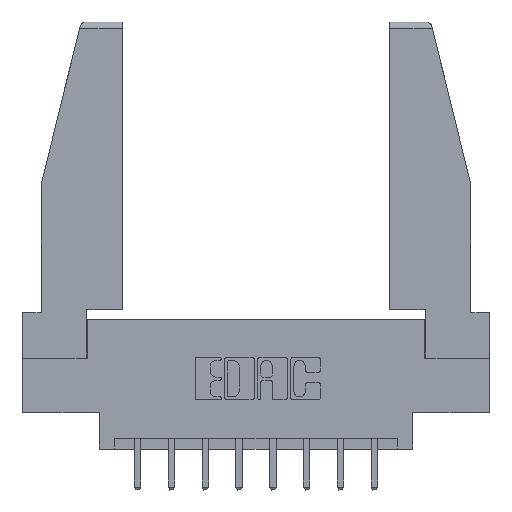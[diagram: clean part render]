
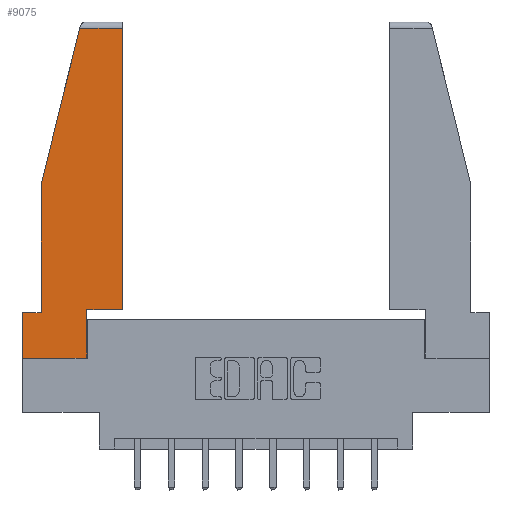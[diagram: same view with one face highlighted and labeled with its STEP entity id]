
A CAD part, top view. The second image highlights one B-rep face of the part: STEP entity #9075.
In plain terms, the highlighted planar face has unit normal (0, 0, 1).
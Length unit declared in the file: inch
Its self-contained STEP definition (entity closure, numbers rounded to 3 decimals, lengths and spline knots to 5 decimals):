
#29 = VERTEX_POINT ( 'NONE', #10967 ) ;
#134 = DIRECTION ( 'NONE',  ( 0., -1., 0. ) ) ;
#291 = ORIENTED_EDGE ( 'NONE', *, *, #1685, .T. ) ;
#474 = LINE ( 'NONE', #6805, #2551 ) ;
#528 = VERTEX_POINT ( 'NONE', #4427 ) ;
#845 = VECTOR ( 'NONE', #8664, 39.37008 ) ;
#1119 = VECTOR ( 'NONE', #6566, 39.37008 ) ;
#1157 = DIRECTION ( 'NONE',  ( 0., 1., 0. ) ) ;
#1420 = VERTEX_POINT ( 'NONE', #6144 ) ;
#1426 = VECTOR ( 'NONE', #8244, 39.37008 ) ;
#1634 = ORIENTED_EDGE ( 'NONE', *, *, #9630, .T. ) ;
#1685 = EDGE_CURVE ( 'NONE', #1420, #528, #12575, .T. ) ;
#1731 = EDGE_CURVE ( 'NONE', #9567, #5478, #4646, .T. ) ;
#1745 = CARTESIAN_POINT ( 'NONE',  ( 0., 0.21, 0. ) ) ;
#2107 = DIRECTION ( 'NONE',  ( 0., 0., 1. ) ) ;
#2132 = LINE ( 'NONE', #12660, #845 ) ;
#2157 = ORIENTED_EDGE ( 'NONE', *, *, #1731, .T. ) ;
#2300 = DIRECTION ( 'NONE',  ( 0., 1., 0. ) ) ;
#2551 = VECTOR ( 'NONE', #7887, 39.37008 ) ;
#2657 = EDGE_CURVE ( 'NONE', #5478, #3469, #474, .T. ) ;
#2764 = ORIENTED_EDGE ( 'NONE', *, *, #2977, .T. ) ;
#2782 = LINE ( 'NONE', #5480, #9214 ) ;
#2977 = EDGE_CURVE ( 'NONE', #3469, #12307, #10913, .T. ) ;
#3406 = LINE ( 'NONE', #8216, #6632 ) ;
#3469 = VERTEX_POINT ( 'NONE', #1745 ) ;
#4027 = PLANE ( 'NONE',  #12430 ) ;
#4427 = CARTESIAN_POINT ( 'NONE',  ( 0.297, 0.223, 0. ) ) ;
#4522 = CARTESIAN_POINT ( 'NONE',  ( 0.086, 0.8, 0. ) ) ;
#4646 = LINE ( 'NONE', #4522, #1119 ) ;
#4932 = ORIENTED_EDGE ( 'NONE', *, *, #8608, .T. ) ;
#5478 = VERTEX_POINT ( 'NONE', #9220 ) ;
#5480 = CARTESIAN_POINT ( 'NONE',  ( 0.271, 1.55, 0. ) ) ;
#5542 = CARTESIAN_POINT ( 'NONE',  ( 0.086, 0.8, 0. ) ) ;
#5574 = CARTESIAN_POINT ( 'NONE',  ( 0.461, 0.223, 0. ) ) ;
#5576 = CARTESIAN_POINT ( 'NONE',  ( 0., 0., 0. ) ) ;
#5590 = EDGE_CURVE ( 'NONE', #29, #9567, #2782, .T. ) ;
#5676 = VERTEX_POINT ( 'NONE', #11947 ) ;
#5790 = VECTOR ( 'NONE', #134, 39.37008 ) ;
#5945 = VECTOR ( 'NONE', #6618, 39.37008 ) ;
#6112 = CARTESIAN_POINT ( 'NONE',  ( 0.297, 0., 0. ) ) ;
#6144 = CARTESIAN_POINT ( 'NONE',  ( 0.297, 0., 0. ) ) ;
#6246 = DIRECTION ( 'NONE',  ( 1., 0., 0. ) ) ;
#6270 = EDGE_LOOP ( 'NONE', ( #4932, #11247, #13326, #2157, #13142, #2764, #1634, #291, #10011 ) ) ;
#6566 = DIRECTION ( 'NONE',  ( 0., -1., 0. ) ) ;
#6618 = DIRECTION ( 'NONE',  ( 1., 0., 0. ) ) ;
#6632 = VECTOR ( 'NONE', #1157, 39.37008 ) ;
#6805 = CARTESIAN_POINT ( 'NONE',  ( 0., 0.21, 0. ) ) ;
#6829 = DIRECTION ( 'NONE',  ( -0.239, -0.971, 0. ) ) ;
#6931 = EDGE_CURVE ( 'NONE', #5676, #29, #2132, .T. ) ;
#7236 = CARTESIAN_POINT ( 'NONE',  ( 0.297, 0.223, 0. ) ) ;
#7254 = FACE_OUTER_BOUND ( 'NONE', #6270, .T. ) ;
#7689 = VERTEX_POINT ( 'NONE', #5574 ) ;
#7887 = DIRECTION ( 'NONE',  ( -1., 0., 0. ) ) ;
#8152 = LINE ( 'NONE', #5576, #5945 ) ;
#8216 = CARTESIAN_POINT ( 'NONE',  ( 0.461, 0.223, 0. ) ) ;
#8244 = DIRECTION ( 'NONE',  ( 1., 0., 0. ) ) ;
#8349 = VECTOR ( 'NONE', #2300, 39.37008 ) ;
#8608 = EDGE_CURVE ( 'NONE', #7689, #5676, #3406, .T. ) ;
#8664 = DIRECTION ( 'NONE',  ( -1., 0., 0. ) ) ;
#9009 = CARTESIAN_POINT ( 'NONE',  ( 0., 0., 0. ) ) ;
#9075 = ADVANCED_FACE ( 'NONE', ( #7254 ), #4027, .T. ) ;
#9214 = VECTOR ( 'NONE', #6829, 39.37008 ) ;
#9220 = CARTESIAN_POINT ( 'NONE',  ( 0.086, 0.21, 0. ) ) ;
#9459 = CARTESIAN_POINT ( 'NONE',  ( 0., 0., 0. ) ) ;
#9567 = VERTEX_POINT ( 'NONE', #5542 ) ;
#9630 = EDGE_CURVE ( 'NONE', #12307, #1420, #8152, .T. ) ;
#10011 = ORIENTED_EDGE ( 'NONE', *, *, #11203, .T. ) ;
#10468 = LINE ( 'NONE', #7236, #1426 ) ;
#10913 = LINE ( 'NONE', #11408, #5790 ) ;
#10967 = CARTESIAN_POINT ( 'NONE',  ( 0.2636, 1.52, 0. ) ) ;
#11203 = EDGE_CURVE ( 'NONE', #528, #7689, #10468, .T. ) ;
#11247 = ORIENTED_EDGE ( 'NONE', *, *, #6931, .T. ) ;
#11408 = CARTESIAN_POINT ( 'NONE',  ( 0., 0.21, 0. ) ) ;
#11947 = CARTESIAN_POINT ( 'NONE',  ( 0.461, 1.52, 0. ) ) ;
#12307 = VERTEX_POINT ( 'NONE', #9009 ) ;
#12430 = AXIS2_PLACEMENT_3D ( 'NONE', #9459, #2107, #6246 ) ;
#12575 = LINE ( 'NONE', #6112, #8349 ) ;
#12660 = CARTESIAN_POINT ( 'NONE',  ( 0., 1.52, 0. ) ) ;
#13142 = ORIENTED_EDGE ( 'NONE', *, *, #2657, .T. ) ;
#13326 = ORIENTED_EDGE ( 'NONE', *, *, #5590, .T. ) ;
